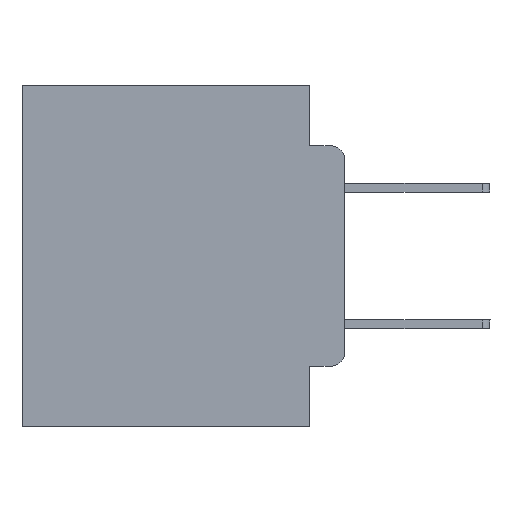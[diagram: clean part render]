
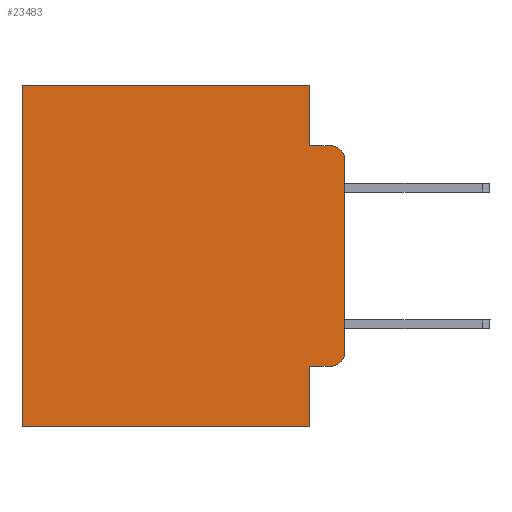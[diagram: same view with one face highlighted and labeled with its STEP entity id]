
A CAD part, left-side view. The second image highlights one B-rep face of the part: STEP entity #23483.
In plain terms, the highlighted planar face has unit normal (-1, 0, 0).
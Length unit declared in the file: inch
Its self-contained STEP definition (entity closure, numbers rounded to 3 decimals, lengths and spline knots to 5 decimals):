
#103 = CARTESIAN_POINT ( 'NONE',  ( 0.298, 0., 0. ) ) ;
#925 = CARTESIAN_POINT ( 'NONE',  ( 0.298, 0.051, -0.4115 ) ) ;
#1653 = ORIENTED_EDGE ( 'NONE', *, *, #10139, .F. ) ;
#2395 = VERTEX_POINT ( 'NONE', #20011 ) ;
#2539 = LINE ( 'NONE', #13205, #22270 ) ;
#2768 = LINE ( 'NONE', #12977, #25020 ) ;
#2913 = AXIS2_PLACEMENT_3D ( 'NONE', #15681, #13741, #9497 ) ;
#3208 = VECTOR ( 'NONE', #21970, 39.37008 ) ;
#3430 = VERTEX_POINT ( 'NONE', #24370 ) ;
#3987 = VERTEX_POINT ( 'NONE', #17443 ) ;
#4160 = CARTESIAN_POINT ( 'NONE',  ( 0.298, 0.051, 0. ) ) ;
#4885 = DIRECTION ( 'NONE',  ( 0., 0., -1. ) ) ;
#4990 = ORIENTED_EDGE ( 'NONE', *, *, #8265, .F. ) ;
#4994 = VERTEX_POINT ( 'NONE', #8305 ) ;
#5096 = CARTESIAN_POINT ( 'NONE',  ( 0.298, 0., 0. ) ) ;
#5338 = CARTESIAN_POINT ( 'NONE',  ( 0.298, 0.051, -0.0885 ) ) ;
#5547 = CIRCLE ( 'NONE', #5915, 0.02 ) ;
#5915 = AXIS2_PLACEMENT_3D ( 'NONE', #17901, #18084, #10115 ) ;
#5964 = EDGE_CURVE ( 'NONE', #25614, #2395, #2539, .T. ) ;
#6051 = VECTOR ( 'NONE', #4885, 39.37008 ) ;
#6368 = LINE ( 'NONE', #12000, #18472 ) ;
#6401 = VERTEX_POINT ( 'NONE', #24482 ) ;
#7445 = EDGE_CURVE ( 'NONE', #3987, #16429, #5547, .T. ) ;
#7488 = EDGE_CURVE ( 'NONE', #17318, #16429, #13520, .T. ) ;
#7595 = VECTOR ( 'NONE', #13274, 39.37008 ) ;
#7659 = CARTESIAN_POINT ( 'NONE',  ( 0.298, 0.051, -0.4115 ) ) ;
#7801 = CARTESIAN_POINT ( 'NONE',  ( 0.298, 0.051, -0.0885 ) ) ;
#7995 = LINE ( 'NONE', #13069, #6051 ) ;
#8265 = EDGE_CURVE ( 'NONE', #20556, #6401, #19532, .T. ) ;
#8302 = PLANE ( 'NONE',  #17351 ) ;
#8305 = CARTESIAN_POINT ( 'NONE',  ( 0.298, 0., -0.3915 ) ) ;
#9278 = DIRECTION ( 'NONE',  ( 0., 0., -1. ) ) ;
#9497 = DIRECTION ( 'NONE',  ( 0., 0., -1. ) ) ;
#9579 = CARTESIAN_POINT ( 'NONE',  ( 0.298, 0.473, 0. ) ) ;
#10115 = DIRECTION ( 'NONE',  ( 0., 0., -1. ) ) ;
#10139 = EDGE_CURVE ( 'NONE', #16708, #17318, #7995, .T. ) ;
#10415 = EDGE_CURVE ( 'NONE', #20556, #3430, #13692, .T. ) ;
#10417 = EDGE_CURVE ( 'NONE', #16708, #25614, #6368, .T. ) ;
#11799 = EDGE_CURVE ( 'NONE', #3987, #4994, #23797, .T. ) ;
#12000 = CARTESIAN_POINT ( 'NONE',  ( 0.298, 0., 0. ) ) ;
#12382 = DIRECTION ( 'NONE',  ( 1., 0., 0. ) ) ;
#12467 = EDGE_CURVE ( 'NONE', #6401, #2395, #2768, .T. ) ;
#12977 = CARTESIAN_POINT ( 'NONE',  ( 0.298, 0., -0.5 ) ) ;
#13069 = CARTESIAN_POINT ( 'NONE',  ( 0.298, 0.051, 0. ) ) ;
#13205 = CARTESIAN_POINT ( 'NONE',  ( 0.298, 0.473, 0. ) ) ;
#13274 = DIRECTION ( 'NONE',  ( 0., 0., -1. ) ) ;
#13520 = LINE ( 'NONE', #7801, #19216 ) ;
#13692 = LINE ( 'NONE', #7659, #3208 ) ;
#13711 = ORIENTED_EDGE ( 'NONE', *, *, #7445, .T. ) ;
#13741 = DIRECTION ( 'NONE',  ( -1., 0., 0. ) ) ;
#14317 = EDGE_CURVE ( 'NONE', #3430, #4994, #22578, .T. ) ;
#15681 = CARTESIAN_POINT ( 'NONE',  ( 0.298, 0.02, -0.3915 ) ) ;
#15717 = ORIENTED_EDGE ( 'NONE', *, *, #14317, .T. ) ;
#16031 = DIRECTION ( 'NONE',  ( 0., -1., 0. ) ) ;
#16429 = VERTEX_POINT ( 'NONE', #19540 ) ;
#16708 = VERTEX_POINT ( 'NONE', #4160 ) ;
#17318 = VERTEX_POINT ( 'NONE', #5338 ) ;
#17351 = AXIS2_PLACEMENT_3D ( 'NONE', #103, #12382, #18421 ) ;
#17443 = CARTESIAN_POINT ( 'NONE',  ( 0.298, 0., -0.1085 ) ) ;
#17901 = CARTESIAN_POINT ( 'NONE',  ( 0.298, 0.02, -0.1085 ) ) ;
#18084 = DIRECTION ( 'NONE',  ( -1., 0., 0. ) ) ;
#18421 = DIRECTION ( 'NONE',  ( 0., 0., -1. ) ) ;
#18472 = VECTOR ( 'NONE', #26197, 39.37008 ) ;
#19027 = ORIENTED_EDGE ( 'NONE', *, *, #10415, .T. ) ;
#19216 = VECTOR ( 'NONE', #16031, 39.37008 ) ;
#19419 = DIRECTION ( 'NONE',  ( 0., 0., -1. ) ) ;
#19420 = ORIENTED_EDGE ( 'NONE', *, *, #10417, .T. ) ;
#19532 = LINE ( 'NONE', #21484, #20833 ) ;
#19540 = CARTESIAN_POINT ( 'NONE',  ( 0.298, 0.02, -0.0885 ) ) ;
#20011 = CARTESIAN_POINT ( 'NONE',  ( 0.298, 0.473, -0.5 ) ) ;
#20232 = ORIENTED_EDGE ( 'NONE', *, *, #5964, .T. ) ;
#20261 = ORIENTED_EDGE ( 'NONE', *, *, #12467, .F. ) ;
#20556 = VERTEX_POINT ( 'NONE', #925 ) ;
#20833 = VECTOR ( 'NONE', #9278, 39.37008 ) ;
#21484 = CARTESIAN_POINT ( 'NONE',  ( 0.298, 0.051, 0. ) ) ;
#21970 = DIRECTION ( 'NONE',  ( 0., -1., 0. ) ) ;
#22270 = VECTOR ( 'NONE', #19419, 39.37008 ) ;
#22578 = CIRCLE ( 'NONE', #2913, 0.02 ) ;
#22780 = ORIENTED_EDGE ( 'NONE', *, *, #11799, .F. ) ;
#23019 = EDGE_LOOP ( 'NONE', ( #22780, #13711, #26160, #1653, #19420, #20232, #20261, #4990, #19027, #15717 ) ) ;
#23483 = ADVANCED_FACE ( 'NONE', ( #23993 ), #8302, .F. ) ;
#23797 = LINE ( 'NONE', #5096, #7595 ) ;
#23993 = FACE_OUTER_BOUND ( 'NONE', #23019, .T. ) ;
#24370 = CARTESIAN_POINT ( 'NONE',  ( 0.298, 0.02, -0.4115 ) ) ;
#24482 = CARTESIAN_POINT ( 'NONE',  ( 0.298, 0.051, -0.5 ) ) ;
#25020 = VECTOR ( 'NONE', #25233, 39.37008 ) ;
#25233 = DIRECTION ( 'NONE',  ( 0., 1., 0. ) ) ;
#25614 = VERTEX_POINT ( 'NONE', #9579 ) ;
#26160 = ORIENTED_EDGE ( 'NONE', *, *, #7488, .F. ) ;
#26197 = DIRECTION ( 'NONE',  ( 0., 1., 0. ) ) ;
